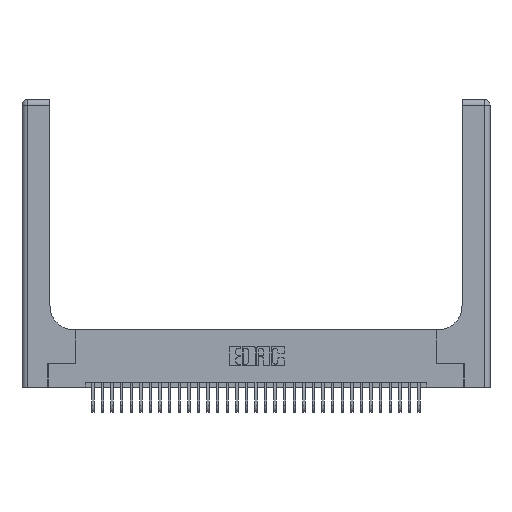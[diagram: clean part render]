
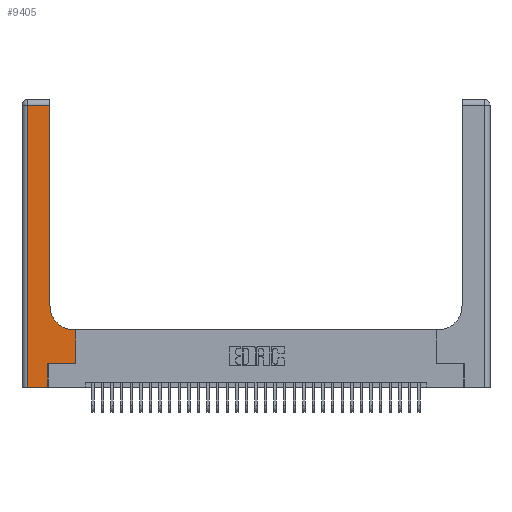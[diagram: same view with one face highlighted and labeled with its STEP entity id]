
A CAD part, top view. The second image highlights one B-rep face of the part: STEP entity #9405.
In plain terms, the highlighted planar face has unit normal (0, 0, 1).
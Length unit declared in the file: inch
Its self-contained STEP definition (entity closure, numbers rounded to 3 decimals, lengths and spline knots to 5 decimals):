
#572 = VERTEX_POINT ( 'NONE', #17723 ) ;
#883 = DIRECTION ( 'NONE',  ( 0., -1., 0. ) ) ;
#1268 = LINE ( 'NONE', #27909, #15020 ) ;
#2136 = CARTESIAN_POINT ( 'NONE',  ( 0.269, 0., 0.37 ) ) ;
#2511 = PLANE ( 'NONE',  #25817 ) ;
#2559 = FACE_OUTER_BOUND ( 'NONE', #21969, .T. ) ;
#2847 = CARTESIAN_POINT ( 'NONE',  ( 0.5415, 0.85, 0.37 ) ) ;
#3182 = EDGE_CURVE ( 'NONE', #8484, #3398, #1268, .T. ) ;
#3253 = VERTEX_POINT ( 'NONE', #9254 ) ;
#3398 = VERTEX_POINT ( 'NONE', #23333 ) ;
#4626 = VECTOR ( 'NONE', #4916, 39.37008 ) ;
#4916 = DIRECTION ( 'NONE',  ( 0., 1., 0. ) ) ;
#5207 = DIRECTION ( 'NONE',  ( 1., 0., 0. ) ) ;
#5252 = CARTESIAN_POINT ( 'NONE',  ( 0.5415, 0.6, 0.37 ) ) ;
#5292 = DIRECTION ( 'NONE',  ( 0., 0., -1. ) ) ;
#5614 = DIRECTION ( 'NONE',  ( 1., 0., 0. ) ) ;
#5889 = LINE ( 'NONE', #21595, #34797 ) ;
#6020 = CARTESIAN_POINT ( 'NONE',  ( 0.06, 0., 0.37 ) ) ;
#6173 = ORIENTED_EDGE ( 'NONE', *, *, #26174, .T. ) ;
#6505 = VERTEX_POINT ( 'NONE', #25094 ) ;
#6788 = ORIENTED_EDGE ( 'NONE', *, *, #7258, .T. ) ;
#7101 = CARTESIAN_POINT ( 'NONE',  ( 0.5585, 0.25, 0.37 ) ) ;
#7258 = EDGE_CURVE ( 'NONE', #22236, #3253, #12211, .T. ) ;
#8041 = VERTEX_POINT ( 'NONE', #5252 ) ;
#8484 = VERTEX_POINT ( 'NONE', #26430 ) ;
#8681 = CARTESIAN_POINT ( 'NONE',  ( 0.2915, 0.6, 0.37 ) ) ;
#8857 = EDGE_CURVE ( 'NONE', #3253, #8041, #20640, .T. ) ;
#9254 = CARTESIAN_POINT ( 'NONE',  ( 0.5585, 0.6, 0.37 ) ) ;
#9405 = ADVANCED_FACE ( 'NONE', ( #2559 ), #2511, .F. ) ;
#10947 = ORIENTED_EDGE ( 'NONE', *, *, #20143, .T. ) ;
#11185 = AXIS2_PLACEMENT_3D ( 'NONE', #2847, #21996, #5614 ) ;
#11461 = DIRECTION ( 'NONE',  ( -1., 0., 0. ) ) ;
#11525 = CARTESIAN_POINT ( 'NONE',  ( 0.5585, 0.25, 0.37 ) ) ;
#12152 = ORIENTED_EDGE ( 'NONE', *, *, #26566, .T. ) ;
#12211 = LINE ( 'NONE', #7101, #27484 ) ;
#12880 = DIRECTION ( 'NONE',  ( 1., 0., 0. ) ) ;
#13298 = VECTOR ( 'NONE', #12880, 39.37008 ) ;
#13522 = DIRECTION ( 'NONE',  ( 0., 1., 0. ) ) ;
#13730 = ORIENTED_EDGE ( 'NONE', *, *, #8857, .T. ) ;
#14481 = CARTESIAN_POINT ( 'NONE',  ( 0.06, 3., 0.37 ) ) ;
#15020 = VECTOR ( 'NONE', #33353, 39.37008 ) ;
#15185 = EDGE_CURVE ( 'NONE', #6505, #33192, #27231, .T. ) ;
#16107 = EDGE_CURVE ( 'NONE', #3398, #16684, #16495, .T. ) ;
#16212 = CARTESIAN_POINT ( 'NONE',  ( 0., 3., 0.37 ) ) ;
#16495 = LINE ( 'NONE', #14481, #22875 ) ;
#16684 = VERTEX_POINT ( 'NONE', #6020 ) ;
#17723 = CARTESIAN_POINT ( 'NONE',  ( 0.2915, 0.85, 0.37 ) ) ;
#18900 = LINE ( 'NONE', #35051, #24376 ) ;
#20143 = EDGE_CURVE ( 'NONE', #33192, #22236, #5889, .T. ) ;
#20640 = LINE ( 'NONE', #8681, #34149 ) ;
#20998 = CARTESIAN_POINT ( 'NONE',  ( 0., 0., 0.37 ) ) ;
#21595 = CARTESIAN_POINT ( 'NONE',  ( 0.269, 0.25, 0.37 ) ) ;
#21712 = ORIENTED_EDGE ( 'NONE', *, *, #16107, .T. ) ;
#21969 = EDGE_LOOP ( 'NONE', ( #6173, #34835, #21712, #12152, #29614, #10947, #6788, #13730, #31929 ) ) ;
#21996 = DIRECTION ( 'NONE',  ( 0., 0., -1. ) ) ;
#22236 = VERTEX_POINT ( 'NONE', #11525 ) ;
#22875 = VECTOR ( 'NONE', #883, 39.37008 ) ;
#23333 = CARTESIAN_POINT ( 'NONE',  ( 0.06, 2.94, 0.37 ) ) ;
#24376 = VECTOR ( 'NONE', #13522, 39.37008 ) ;
#24380 = DIRECTION ( 'NONE',  ( -1., 0., 0. ) ) ;
#25094 = CARTESIAN_POINT ( 'NONE',  ( 0.269, 0., 0.37 ) ) ;
#25817 = AXIS2_PLACEMENT_3D ( 'NONE', #16212, #5292, #24380 ) ;
#26162 = DIRECTION ( 'NONE',  ( 0., 1., 0. ) ) ;
#26174 = EDGE_CURVE ( 'NONE', #572, #8484, #18900, .T. ) ;
#26430 = CARTESIAN_POINT ( 'NONE',  ( 0.2915, 2.94, 0.37 ) ) ;
#26566 = EDGE_CURVE ( 'NONE', #16684, #6505, #33225, .T. ) ;
#27231 = LINE ( 'NONE', #2136, #4626 ) ;
#27484 = VECTOR ( 'NONE', #26162, 39.37008 ) ;
#27909 = CARTESIAN_POINT ( 'NONE',  ( 0., 2.94, 0.37 ) ) ;
#28646 = EDGE_CURVE ( 'NONE', #8041, #572, #28835, .T. ) ;
#28835 = CIRCLE ( 'NONE', #11185, 0.25 ) ;
#29614 = ORIENTED_EDGE ( 'NONE', *, *, #15185, .T. ) ;
#31453 = CARTESIAN_POINT ( 'NONE',  ( 0.269, 0.25, 0.37 ) ) ;
#31929 = ORIENTED_EDGE ( 'NONE', *, *, #28646, .T. ) ;
#33192 = VERTEX_POINT ( 'NONE', #31453 ) ;
#33225 = LINE ( 'NONE', #20998, #13298 ) ;
#33353 = DIRECTION ( 'NONE',  ( -1., 0., 0. ) ) ;
#34149 = VECTOR ( 'NONE', #11461, 39.37008 ) ;
#34797 = VECTOR ( 'NONE', #5207, 39.37008 ) ;
#34835 = ORIENTED_EDGE ( 'NONE', *, *, #3182, .T. ) ;
#35051 = CARTESIAN_POINT ( 'NONE',  ( 0.2915, 3., 0.37 ) ) ;
